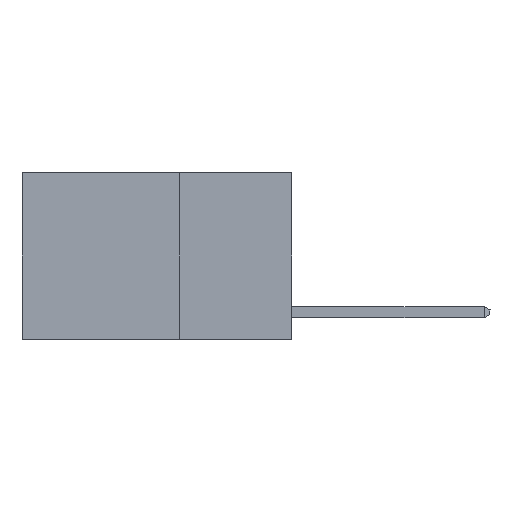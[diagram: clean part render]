
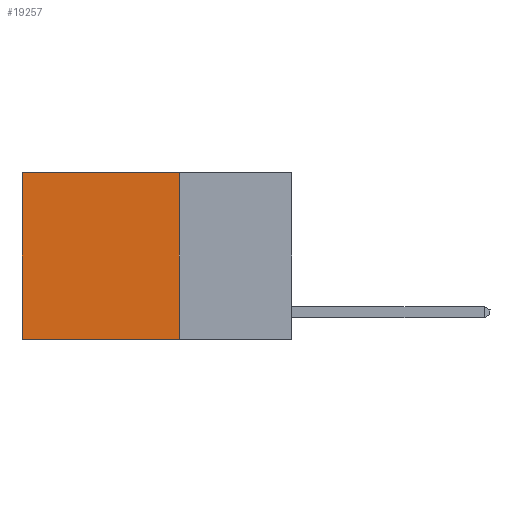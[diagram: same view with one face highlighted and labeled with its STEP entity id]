
A CAD part, left-side view. The second image highlights one B-rep face of the part: STEP entity #19257.
In plain terms, the highlighted planar face has unit normal (-1, 0, 0).
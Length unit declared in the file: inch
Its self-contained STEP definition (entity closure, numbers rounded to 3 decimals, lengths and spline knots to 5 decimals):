
#13 = EDGE_CURVE ( 'NONE', #11708, #5960, #2783, .T. ) ;
#446 = CARTESIAN_POINT ( 'NONE',  ( 0.2625, 0.25, -0.37 ) ) ;
#520 = CARTESIAN_POINT ( 'NONE',  ( 0.2625, 0.25, 0. ) ) ;
#592 = ORIENTED_EDGE ( 'NONE', *, *, #11129, .T. ) ;
#1096 = CARTESIAN_POINT ( 'NONE',  ( 0.2625, 0.25, -0.37 ) ) ;
#1505 = CARTESIAN_POINT ( 'NONE',  ( 0.2625, 0.6, 0. ) ) ;
#1739 = DIRECTION ( 'NONE',  ( 0., 0., -1. ) ) ;
#2159 = DIRECTION ( 'NONE',  ( 0., 0., -1. ) ) ;
#2251 = VERTEX_POINT ( 'NONE', #446 ) ;
#2694 = AXIS2_PLACEMENT_3D ( 'NONE', #10242, #11815, #13533 ) ;
#2783 = LINE ( 'NONE', #14347, #15530 ) ;
#3417 = FACE_OUTER_BOUND ( 'NONE', #13746, .T. ) ;
#3534 = CARTESIAN_POINT ( 'NONE',  ( 0.2625, 0.6, -0.37 ) ) ;
#3790 = ORIENTED_EDGE ( 'NONE', *, *, #12619, .F. ) ;
#5828 = VECTOR ( 'NONE', #10490, 39.37008 ) ;
#5960 = VERTEX_POINT ( 'NONE', #3534 ) ;
#6119 = DIRECTION ( 'NONE',  ( 0., 1., 0. ) ) ;
#7524 = VECTOR ( 'NONE', #1739, 39.37008 ) ;
#9521 = ORIENTED_EDGE ( 'NONE', *, *, #13, .T. ) ;
#9701 = VERTEX_POINT ( 'NONE', #13062 ) ;
#10242 = CARTESIAN_POINT ( 'NONE',  ( 0.2625, 0.25, 0. ) ) ;
#10490 = DIRECTION ( 'NONE',  ( 0., 1., 0. ) ) ;
#11129 = EDGE_CURVE ( 'NONE', #9701, #11708, #11441, .T. ) ;
#11441 = LINE ( 'NONE', #15584, #14666 ) ;
#11708 = VERTEX_POINT ( 'NONE', #1505 ) ;
#11815 = DIRECTION ( 'NONE',  ( 1., 0., 0. ) ) ;
#12270 = EDGE_CURVE ( 'NONE', #2251, #5960, #18247, .T. ) ;
#12619 = EDGE_CURVE ( 'NONE', #9701, #2251, #13090, .T. ) ;
#13062 = CARTESIAN_POINT ( 'NONE',  ( 0.2625, 0.25, 0. ) ) ;
#13090 = LINE ( 'NONE', #520, #7524 ) ;
#13533 = DIRECTION ( 'NONE',  ( 0., 0., -1. ) ) ;
#13746 = EDGE_LOOP ( 'NONE', ( #9521, #14069, #3790, #592 ) ) ;
#14069 = ORIENTED_EDGE ( 'NONE', *, *, #12270, .F. ) ;
#14347 = CARTESIAN_POINT ( 'NONE',  ( 0.2625, 0.6, 0. ) ) ;
#14666 = VECTOR ( 'NONE', #6119, 39.37008 ) ;
#15530 = VECTOR ( 'NONE', #2159, 39.37008 ) ;
#15584 = CARTESIAN_POINT ( 'NONE',  ( 0.2625, 0.25, 0. ) ) ;
#17614 = PLANE ( 'NONE',  #2694 ) ;
#18247 = LINE ( 'NONE', #1096, #5828 ) ;
#19257 = ADVANCED_FACE ( 'NONE', ( #3417 ), #17614, .F. ) ;
